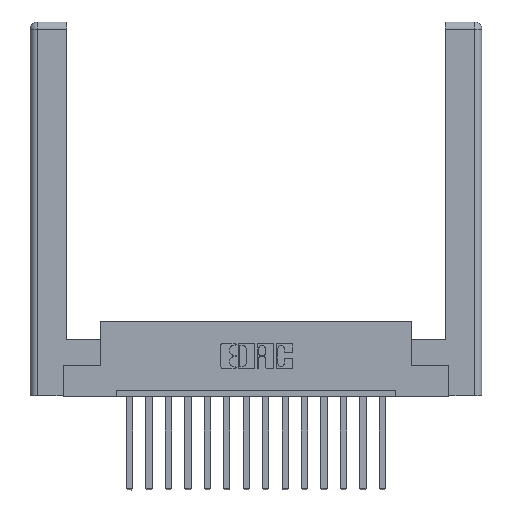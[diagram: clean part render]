
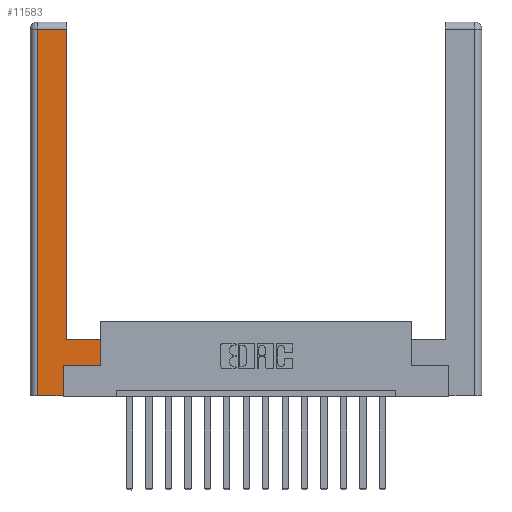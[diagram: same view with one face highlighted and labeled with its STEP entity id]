
A CAD part, top view. The second image highlights one B-rep face of the part: STEP entity #11583.
In plain terms, the highlighted planar face has unit normal (0, 0, 1).
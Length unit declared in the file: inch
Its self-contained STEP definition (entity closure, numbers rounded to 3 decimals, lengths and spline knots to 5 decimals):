
#680 = CARTESIAN_POINT ( 'NONE',  ( 0., 0., 0. ) ) ;
#764 = EDGE_CURVE ( 'NONE', #8931, #14952, #2368, .T. ) ;
#901 = CARTESIAN_POINT ( 'NONE',  ( 0.265, 0., 0. ) ) ;
#1426 = VECTOR ( 'NONE', #8040, 39.37008 ) ;
#1629 = EDGE_LOOP ( 'NONE', ( #3539, #10817, #5656, #12118, #10617, #11009, #4035, #2093 ) ) ;
#1740 = VECTOR ( 'NONE', #12014, 39.37008 ) ;
#1833 = LINE ( 'NONE', #3693, #11003 ) ;
#1929 = CARTESIAN_POINT ( 'NONE',  ( 0.295, 0.45, 0. ) ) ;
#2093 = ORIENTED_EDGE ( 'NONE', *, *, #13337, .T. ) ;
#2368 = LINE ( 'NONE', #7641, #11919 ) ;
#3391 = VERTEX_POINT ( 'NONE', #1929 ) ;
#3438 = CARTESIAN_POINT ( 'NONE',  ( 0.565, 0.245, 0. ) ) ;
#3539 = ORIENTED_EDGE ( 'NONE', *, *, #6726, .T. ) ;
#3693 = CARTESIAN_POINT ( 'NONE',  ( 0.565, 0.45, 0. ) ) ;
#3708 = VERTEX_POINT ( 'NONE', #13020 ) ;
#3966 = LINE ( 'NONE', #6728, #1740 ) ;
#4035 = ORIENTED_EDGE ( 'NONE', *, *, #8927, .T. ) ;
#4374 = CARTESIAN_POINT ( 'NONE',  ( 0.265, 0.245, 0. ) ) ;
#4443 = PLANE ( 'NONE',  #5171 ) ;
#4479 = CARTESIAN_POINT ( 'NONE',  ( 0.0615, 2.94, 0. ) ) ;
#4669 = CARTESIAN_POINT ( 'NONE',  ( 0.0615, 0., 0. ) ) ;
#4956 = VERTEX_POINT ( 'NONE', #11701 ) ;
#5171 = AXIS2_PLACEMENT_3D ( 'NONE', #680, #9624, #13351 ) ;
#5192 = VECTOR ( 'NONE', #5832, 39.37008 ) ;
#5633 = CARTESIAN_POINT ( 'NONE',  ( 0.295, 3., 0. ) ) ;
#5656 = ORIENTED_EDGE ( 'NONE', *, *, #10181, .T. ) ;
#5832 = DIRECTION ( 'NONE',  ( 0., -1., 0. ) ) ;
#5989 = DIRECTION ( 'NONE',  ( 0., 1., 0. ) ) ;
#6726 = EDGE_CURVE ( 'NONE', #3391, #11276, #13606, .T. ) ;
#6728 = CARTESIAN_POINT ( 'NONE',  ( 0.265, 0., 0. ) ) ;
#7641 = CARTESIAN_POINT ( 'NONE',  ( 0.265, 0.245, 0. ) ) ;
#7745 = LINE ( 'NONE', #4479, #7942 ) ;
#7942 = VECTOR ( 'NONE', #14682, 39.37008 ) ;
#7993 = CARTESIAN_POINT ( 'NONE',  ( 0.295, 0.45, 0. ) ) ;
#8040 = DIRECTION ( 'NONE',  ( 0., 1., 0. ) ) ;
#8927 = EDGE_CURVE ( 'NONE', #9622, #3708, #1833, .T. ) ;
#8931 = VERTEX_POINT ( 'NONE', #901 ) ;
#9622 = VERTEX_POINT ( 'NONE', #3438 ) ;
#9624 = DIRECTION ( 'NONE',  ( 0., 0., -1. ) ) ;
#10181 = EDGE_CURVE ( 'NONE', #15829, #4956, #11187, .T. ) ;
#10617 = ORIENTED_EDGE ( 'NONE', *, *, #764, .T. ) ;
#10700 = LINE ( 'NONE', #11800, #13714 ) ;
#10817 = ORIENTED_EDGE ( 'NONE', *, *, #12121, .T. ) ;
#10935 = CARTESIAN_POINT ( 'NONE',  ( 0.295, 2.94, 0. ) ) ;
#11003 = VECTOR ( 'NONE', #5989, 39.37008 ) ;
#11009 = ORIENTED_EDGE ( 'NONE', *, *, #14126, .T. ) ;
#11187 = LINE ( 'NONE', #4669, #5192 ) ;
#11276 = VERTEX_POINT ( 'NONE', #10935 ) ;
#11485 = DIRECTION ( 'NONE',  ( 0., 1., 0. ) ) ;
#11583 = ADVANCED_FACE ( 'NONE', ( #12361 ), #4443, .F. ) ;
#11701 = CARTESIAN_POINT ( 'NONE',  ( 0.0615, 0., 0. ) ) ;
#11800 = CARTESIAN_POINT ( 'NONE',  ( 0.565, 0.245, 0. ) ) ;
#11919 = VECTOR ( 'NONE', #11485, 39.37008 ) ;
#12014 = DIRECTION ( 'NONE',  ( 1., 0., 0. ) ) ;
#12118 = ORIENTED_EDGE ( 'NONE', *, *, #13042, .T. ) ;
#12121 = EDGE_CURVE ( 'NONE', #11276, #15829, #7745, .T. ) ;
#12361 = FACE_OUTER_BOUND ( 'NONE', #1629, .T. ) ;
#13020 = CARTESIAN_POINT ( 'NONE',  ( 0.565, 0.45, 0. ) ) ;
#13042 = EDGE_CURVE ( 'NONE', #4956, #8931, #3966, .T. ) ;
#13337 = EDGE_CURVE ( 'NONE', #3708, #3391, #14198, .T. ) ;
#13351 = DIRECTION ( 'NONE',  ( -1., 0., 0. ) ) ;
#13375 = CARTESIAN_POINT ( 'NONE',  ( 0.0615, 2.94, 0. ) ) ;
#13606 = LINE ( 'NONE', #5633, #1426 ) ;
#13714 = VECTOR ( 'NONE', #15746, 39.37008 ) ;
#13815 = VECTOR ( 'NONE', #14452, 39.37008 ) ;
#14126 = EDGE_CURVE ( 'NONE', #14952, #9622, #10700, .T. ) ;
#14198 = LINE ( 'NONE', #7993, #13815 ) ;
#14452 = DIRECTION ( 'NONE',  ( -1., 0., 0. ) ) ;
#14682 = DIRECTION ( 'NONE',  ( -1., 0., 0. ) ) ;
#14952 = VERTEX_POINT ( 'NONE', #4374 ) ;
#15746 = DIRECTION ( 'NONE',  ( 1., 0., 0. ) ) ;
#15829 = VERTEX_POINT ( 'NONE', #13375 ) ;
